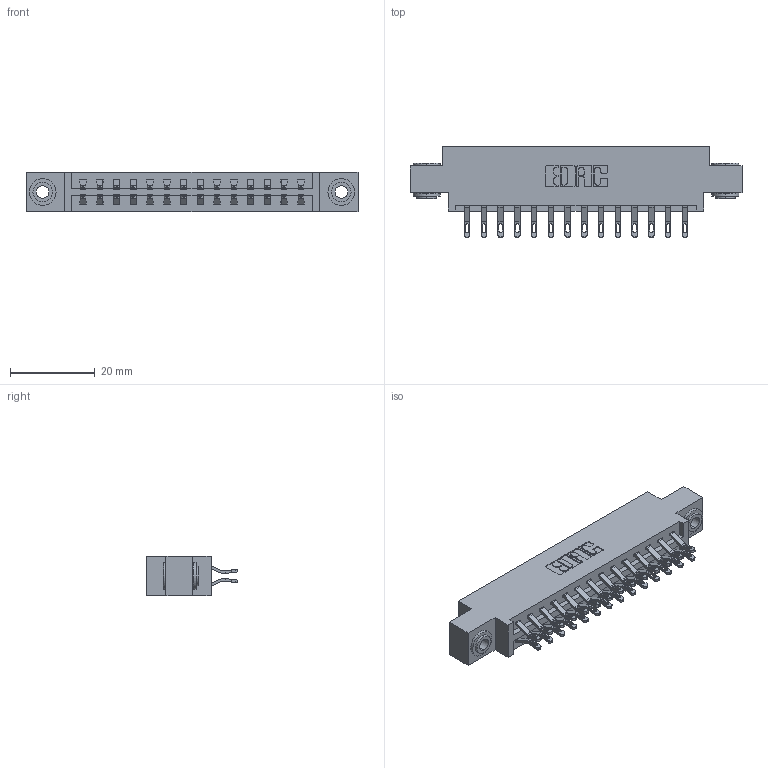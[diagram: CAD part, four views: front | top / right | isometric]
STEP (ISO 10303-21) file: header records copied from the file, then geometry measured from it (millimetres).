
FILE_DESCRIPTION (( 'STEP AP203' ), '1' );
FILE_NAME ('387-028-555-803.STEP', '2018-09-16T23:01:29', ( '' ), ( '' ), 'SwSTEP 2.0', 'SolidWorks 2016', '' );
FILE_SCHEMA (( 'CONFIG_CONTROL_DESIGN' ));
Length unit declared in the file: inch
Products named in the file (4): 337 Part_0.170 Offset - 0.156 Dia-TH; 345-292-001_555 Tail; 345-250-002_345-250-002-102; 387-028-555-803
Assembly tree (31 placements, depth 2):
  387-028-555-803
    337 Part_0.170 Offset - 0.156 Dia-TH
    345-292-001_555 Tail  x28
    345-250-002_345-250-002-102  x2
Bounding box: 78.49 x 21.47 x 9.4 mm (x, y, z)
Volume: 7881.9 mm3; surface area: 9276.8 mm2
Topology: 31 solids, 31 shells, 1836 faces, 5691 edges, 3790 vertices
Faces by surface type: plane 1092, cylinder 736, cone 8
Entity records: 15584 total; most frequent: CARTESIAN_POINT 2659, ORIENTED_EDGE 2558, DIRECTION 2317, EDGE_CURVE 1279, VECTOR 1107, LINE 1107, VERTEX_POINT 850, AXIS2_PLACEMENT_3D 605
